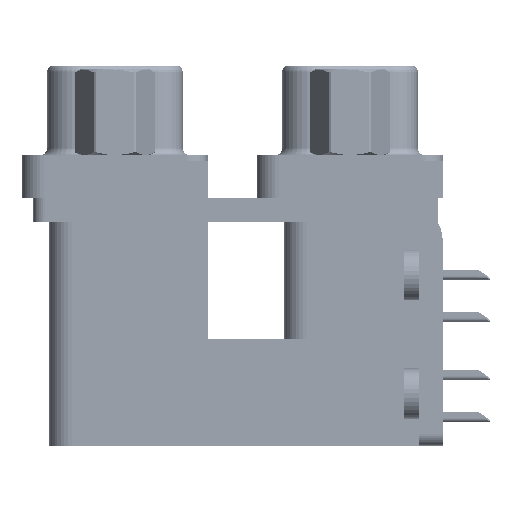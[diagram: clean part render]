
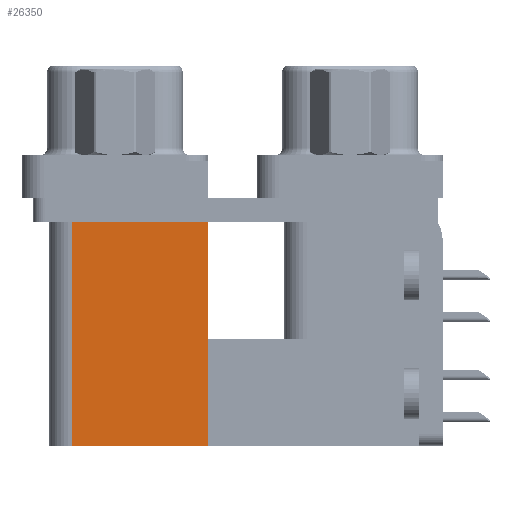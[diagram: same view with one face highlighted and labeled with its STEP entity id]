
A CAD part, left-side view. The second image highlights one B-rep face of the part: STEP entity #26350.
In plain terms, the highlighted planar face has unit normal (-1, 0, 0).
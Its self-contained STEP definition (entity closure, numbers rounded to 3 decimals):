
#8665 = EDGE_CURVE ( 'NONE', #20737, #12897, #29271, .T. ) ;
#11065 = CARTESIAN_POINT ( 'NONE',  ( 3.79, 9.6, -19.2 ) ) ;
#11509 = AXIS2_PLACEMENT_3D ( 'NONE', #35339, #48568, #13572 ) ;
#11857 = CARTESIAN_POINT ( 'NONE',  ( 3.79, 9.6, -19.2 ) ) ;
#12897 = VERTEX_POINT ( 'NONE', #18811 ) ;
#13133 = ORIENTED_EDGE ( 'NONE', *, *, #37841, .T. ) ;
#13572 = DIRECTION ( 'NONE',  ( 0., 0., -1. ) ) ;
#13824 = VECTOR ( 'NONE', #40458, 1000. ) ;
#14177 = EDGE_CURVE ( 'NONE', #39480, #20737, #35331, .T. ) ;
#18556 = PLANE ( 'NONE',  #11509 ) ;
#18811 = CARTESIAN_POINT ( 'NONE',  ( 3.79, 18.8, -2.5 ) ) ;
#20737 = VERTEX_POINT ( 'NONE', #22452 ) ;
#22251 = LINE ( 'NONE', #22539, #13824 ) ;
#22452 = CARTESIAN_POINT ( 'NONE',  ( 3.79, 18.8, -19.2 ) ) ;
#22539 = CARTESIAN_POINT ( 'NONE',  ( 3.79, 9.6, -2.5 ) ) ;
#26350 = ADVANCED_FACE ( 'NONE', ( #44720 ), #18556, .F. ) ;
#26591 = VECTOR ( 'NONE', #53852, 1000. ) ;
#29120 = VECTOR ( 'NONE', #50759, 1000. ) ;
#29271 = LINE ( 'NONE', #37237, #29120 ) ;
#29454 = ORIENTED_EDGE ( 'NONE', *, *, #14177, .F. ) ;
#30234 = EDGE_LOOP ( 'NONE', ( #13133, #38040, #29454, #48239 ) ) ;
#32076 = CARTESIAN_POINT ( 'NONE',  ( 3.79, 9.6, -19.2 ) ) ;
#33716 = DIRECTION ( 'NONE',  ( 0., 0., 1. ) ) ;
#35331 = LINE ( 'NONE', #32076, #26591 ) ;
#35339 = CARTESIAN_POINT ( 'NONE',  ( 3.79, 9.6, -19.2 ) ) ;
#36964 = LINE ( 'NONE', #11065, #49160 ) ;
#37237 = CARTESIAN_POINT ( 'NONE',  ( 3.79, 18.8, -19.2 ) ) ;
#37841 = EDGE_CURVE ( 'NONE', #39838, #12897, #22251, .T. ) ;
#38040 = ORIENTED_EDGE ( 'NONE', *, *, #8665, .F. ) ;
#39480 = VERTEX_POINT ( 'NONE', #11857 ) ;
#39838 = VERTEX_POINT ( 'NONE', #50929 ) ;
#40458 = DIRECTION ( 'NONE',  ( 0., 1., 0. ) ) ;
#44720 = FACE_OUTER_BOUND ( 'NONE', #30234, .T. ) ;
#47308 = EDGE_CURVE ( 'NONE', #39480, #39838, #36964, .T. ) ;
#48239 = ORIENTED_EDGE ( 'NONE', *, *, #47308, .T. ) ;
#48568 = DIRECTION ( 'NONE',  ( 1., 0., 0. ) ) ;
#49160 = VECTOR ( 'NONE', #33716, 1000. ) ;
#50759 = DIRECTION ( 'NONE',  ( 0., 0., 1. ) ) ;
#50929 = CARTESIAN_POINT ( 'NONE',  ( 3.79, 9.6, -2.5 ) ) ;
#53852 = DIRECTION ( 'NONE',  ( 0., 1., 0. ) ) ;
